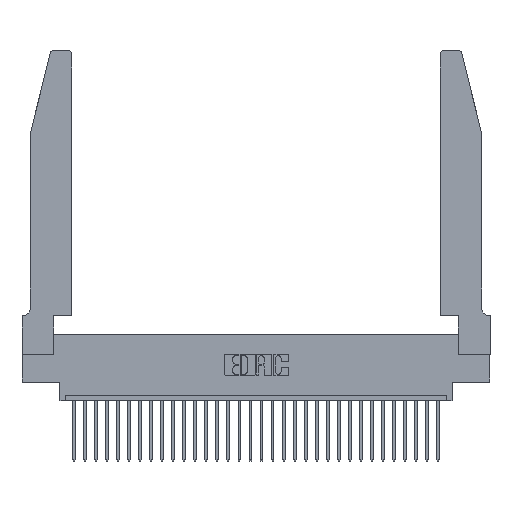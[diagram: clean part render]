
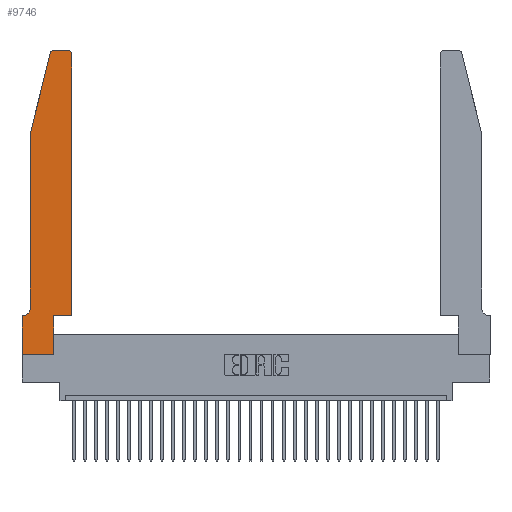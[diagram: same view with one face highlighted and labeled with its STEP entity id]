
A CAD part, top view. The second image highlights one B-rep face of the part: STEP entity #9746.
In plain terms, the highlighted planar face has unit normal (0, 0, 1).
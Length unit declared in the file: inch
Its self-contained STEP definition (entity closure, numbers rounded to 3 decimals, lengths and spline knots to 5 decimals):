
#466 = ORIENTED_EDGE ( 'NONE', *, *, #23060, .T. ) ;
#495 = LINE ( 'NONE', #10333, #16926 ) ;
#666 = EDGE_CURVE ( 'NONE', #22471, #14135, #19007, .T. ) ;
#823 = DIRECTION ( 'NONE',  ( 0., 0., 1. ) ) ;
#882 = CARTESIAN_POINT ( 'NONE',  ( 0.0055, 0.42, 0.37 ) ) ;
#921 = CARTESIAN_POINT ( 'NONE',  ( 0.4505, 0.35, 0.37 ) ) ;
#923 = CIRCLE ( 'NONE', #11426, 0.07 ) ;
#1964 = DIRECTION ( 'NONE',  ( -1., 0., 0. ) ) ;
#2092 = FACE_OUTER_BOUND ( 'NONE', #16629, .T. ) ;
#2334 = LINE ( 'NONE', #25348, #21036 ) ;
#3247 = ORIENTED_EDGE ( 'NONE', *, *, #17493, .T. ) ;
#3306 = DIRECTION ( 'NONE',  ( 0., 0., -1. ) ) ;
#3320 = LINE ( 'NONE', #31052, #11409 ) ;
#3638 = CIRCLE ( 'NONE', #31462, 0.03 ) ;
#4845 = EDGE_CURVE ( 'NONE', #21478, #17619, #3320, .T. ) ;
#5128 = VERTEX_POINT ( 'NONE', #25123 ) ;
#5442 = DIRECTION ( 'NONE',  ( 1., 0., 0. ) ) ;
#6212 = CARTESIAN_POINT ( 'NONE',  ( 0.0055, 0.35, 0.37 ) ) ;
#6575 = LINE ( 'NONE', #21405, #11915 ) ;
#6999 = VERTEX_POINT ( 'NONE', #28841 ) ;
#7010 = VECTOR ( 'NONE', #1964, 39.37008 ) ;
#7114 = ORIENTED_EDGE ( 'NONE', *, *, #8057, .T. ) ;
#7281 = VERTEX_POINT ( 'NONE', #6212 ) ;
#7607 = LINE ( 'NONE', #17607, #24459 ) ;
#8057 = EDGE_CURVE ( 'NONE', #14135, #21478, #3638, .T. ) ;
#8630 = CARTESIAN_POINT ( 'NONE',  ( 0.0755, 2., 0.37 ) ) ;
#8778 = CARTESIAN_POINT ( 'NONE',  ( 0.2865, 0.35, 0.37 ) ) ;
#9354 = CARTESIAN_POINT ( 'NONE',  ( 0.25487, 2.72718, 0.37 ) ) ;
#9600 = CARTESIAN_POINT ( 'NONE',  ( 0.4505, 2.72, 0.37 ) ) ;
#9746 = ADVANCED_FACE ( 'NONE', ( #2092 ), #12983, .T. ) ;
#10236 = CARTESIAN_POINT ( 'NONE',  ( 0.284, 2.72, 0.37 ) ) ;
#10333 = CARTESIAN_POINT ( 'NONE',  ( 0., 0., 0.37 ) ) ;
#10553 = DIRECTION ( 'NONE',  ( 1., 0., 0. ) ) ;
#10616 = DIRECTION ( 'NONE',  ( -0.239, -0.971, 0. ) ) ;
#10654 = LINE ( 'NONE', #23396, #28171 ) ;
#10756 = ORIENTED_EDGE ( 'NONE', *, *, #17233, .T. ) ;
#11165 = ORIENTED_EDGE ( 'NONE', *, *, #19703, .T. ) ;
#11409 = VECTOR ( 'NONE', #18839, 39.37008 ) ;
#11426 = AXIS2_PLACEMENT_3D ( 'NONE', #882, #3306, #17513 ) ;
#11818 = CARTESIAN_POINT ( 'NONE',  ( 0.0755, 0.35, 0.37 ) ) ;
#11915 = VECTOR ( 'NONE', #18854, 39.37008 ) ;
#12387 = VERTEX_POINT ( 'NONE', #8778 ) ;
#12983 = PLANE ( 'NONE',  #26887 ) ;
#13080 = VERTEX_POINT ( 'NONE', #15223 ) ;
#13900 = CARTESIAN_POINT ( 'NONE',  ( 0.284, 2.75, 0.37 ) ) ;
#14135 = VERTEX_POINT ( 'NONE', #9600 ) ;
#14151 = CIRCLE ( 'NONE', #19636, 0.03 ) ;
#15056 = EDGE_CURVE ( 'NONE', #5128, #23836, #495, .T. ) ;
#15223 = CARTESIAN_POINT ( 'NONE',  ( 0.0755, 0.42, 0.37 ) ) ;
#15455 = CARTESIAN_POINT ( 'NONE',  ( 0., 0.35, 0.37 ) ) ;
#15929 = VERTEX_POINT ( 'NONE', #9354 ) ;
#16375 = VECTOR ( 'NONE', #28781, 39.37008 ) ;
#16629 = EDGE_LOOP ( 'NONE', ( #30683, #18419, #17956, #27020, #466, #18714, #20301, #10756, #3247, #11165, #27209, #7114 ) ) ;
#16645 = EDGE_CURVE ( 'NONE', #17619, #15929, #14151, .T. ) ;
#16926 = VECTOR ( 'NONE', #29113, 39.37008 ) ;
#17233 = EDGE_CURVE ( 'NONE', #23836, #6999, #7607, .T. ) ;
#17301 = LINE ( 'NONE', #11818, #7010 ) ;
#17390 = LINE ( 'NONE', #27127, #26571 ) ;
#17493 = EDGE_CURVE ( 'NONE', #6999, #12387, #10654, .T. ) ;
#17513 = DIRECTION ( 'NONE',  ( -1., 0., 0. ) ) ;
#17607 = CARTESIAN_POINT ( 'NONE',  ( 0., 0., 0.37 ) ) ;
#17619 = VERTEX_POINT ( 'NONE', #13900 ) ;
#17646 = CARTESIAN_POINT ( 'NONE',  ( 0.4205, 2.72, 0.37 ) ) ;
#17956 = ORIENTED_EDGE ( 'NONE', *, *, #25029, .T. ) ;
#18419 = ORIENTED_EDGE ( 'NONE', *, *, #16645, .T. ) ;
#18714 = ORIENTED_EDGE ( 'NONE', *, *, #27912, .T. ) ;
#18839 = DIRECTION ( 'NONE',  ( -1., 0., 0. ) ) ;
#18854 = DIRECTION ( 'NONE',  ( 0., -1., 0. ) ) ;
#19007 = LINE ( 'NONE', #24349, #16375 ) ;
#19636 = AXIS2_PLACEMENT_3D ( 'NONE', #10236, #29684, #10553 ) ;
#19703 = EDGE_CURVE ( 'NONE', #12387, #22471, #17390, .T. ) ;
#20301 = ORIENTED_EDGE ( 'NONE', *, *, #15056, .T. ) ;
#21036 = VECTOR ( 'NONE', #10616, 39.37008 ) ;
#21405 = CARTESIAN_POINT ( 'NONE',  ( 0.0755, 2., 0.37 ) ) ;
#21478 = VERTEX_POINT ( 'NONE', #31079 ) ;
#21857 = DIRECTION ( 'NONE',  ( 1., 0., 0. ) ) ;
#22471 = VERTEX_POINT ( 'NONE', #921 ) ;
#22806 = DIRECTION ( 'NONE',  ( 1., 0., 0. ) ) ;
#23060 = EDGE_CURVE ( 'NONE', #13080, #7281, #923, .T. ) ;
#23396 = CARTESIAN_POINT ( 'NONE',  ( 0.2865, 0.35, 0.37 ) ) ;
#23836 = VERTEX_POINT ( 'NONE', #27916 ) ;
#24349 = CARTESIAN_POINT ( 'NONE',  ( 0.4505, 0.35, 0.37 ) ) ;
#24459 = VECTOR ( 'NONE', #5442, 39.37008 ) ;
#24553 = VERTEX_POINT ( 'NONE', #8630 ) ;
#24615 = EDGE_CURVE ( 'NONE', #24553, #13080, #6575, .T. ) ;
#25008 = DIRECTION ( 'NONE',  ( 0., 0., 1. ) ) ;
#25029 = EDGE_CURVE ( 'NONE', #15929, #24553, #2334, .T. ) ;
#25123 = CARTESIAN_POINT ( 'NONE',  ( 0., 0.35, 0.37 ) ) ;
#25348 = CARTESIAN_POINT ( 'NONE',  ( 0.0755, 2., 0.37 ) ) ;
#25845 = DIRECTION ( 'NONE',  ( 0., 1., 0. ) ) ;
#26571 = VECTOR ( 'NONE', #29539, 39.37008 ) ;
#26887 = AXIS2_PLACEMENT_3D ( 'NONE', #15455, #823, #22806 ) ;
#27020 = ORIENTED_EDGE ( 'NONE', *, *, #24615, .T. ) ;
#27127 = CARTESIAN_POINT ( 'NONE',  ( 0.4505, 0.35, 0.37 ) ) ;
#27209 = ORIENTED_EDGE ( 'NONE', *, *, #666, .T. ) ;
#27912 = EDGE_CURVE ( 'NONE', #7281, #5128, #17301, .T. ) ;
#27916 = CARTESIAN_POINT ( 'NONE',  ( 0., 0., 0.37 ) ) ;
#28171 = VECTOR ( 'NONE', #25845, 39.37008 ) ;
#28781 = DIRECTION ( 'NONE',  ( 0., 1., 0. ) ) ;
#28841 = CARTESIAN_POINT ( 'NONE',  ( 0.2865, 0., 0.37 ) ) ;
#29113 = DIRECTION ( 'NONE',  ( 0., -1., 0. ) ) ;
#29539 = DIRECTION ( 'NONE',  ( 1., 0., 0. ) ) ;
#29684 = DIRECTION ( 'NONE',  ( 0., 0., 1. ) ) ;
#30683 = ORIENTED_EDGE ( 'NONE', *, *, #4845, .T. ) ;
#31052 = CARTESIAN_POINT ( 'NONE',  ( 0.2605, 2.75, 0.37 ) ) ;
#31079 = CARTESIAN_POINT ( 'NONE',  ( 0.4205, 2.75, 0.37 ) ) ;
#31462 = AXIS2_PLACEMENT_3D ( 'NONE', #17646, #25008, #21857 ) ;
